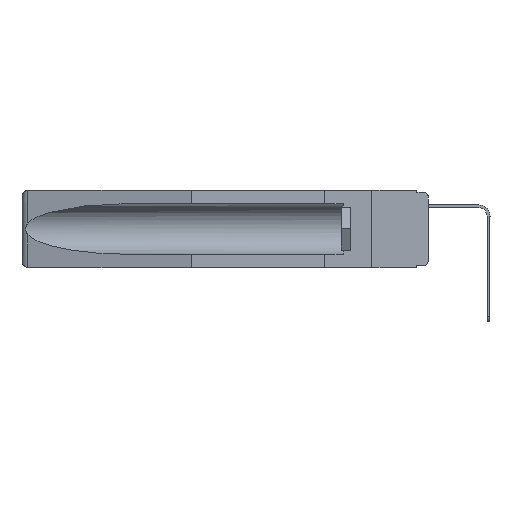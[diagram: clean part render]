
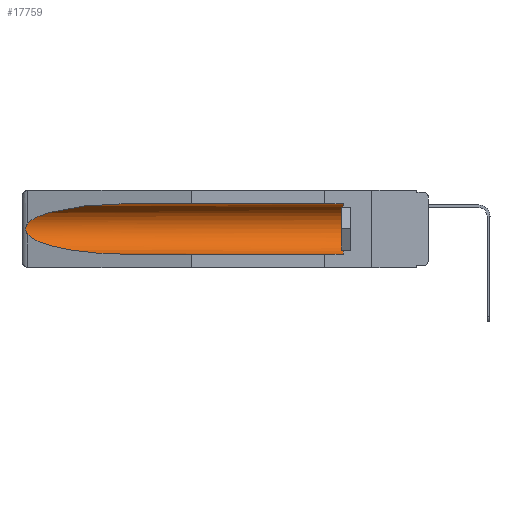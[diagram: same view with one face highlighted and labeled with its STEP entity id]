
A CAD part, left-side view. The second image highlights one B-rep face of the part: STEP entity #17759.
In plain terms, the highlighted cylindrical face has radius 2.857 mm (diameter 5.715 mm), a partial arc.
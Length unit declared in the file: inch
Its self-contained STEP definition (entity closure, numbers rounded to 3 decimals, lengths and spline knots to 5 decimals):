
#1118 = DIRECTION ( 'NONE',  ( 0., 1., 0. ) ) ;
#1183 = CARTESIAN_POINT ( 'NONE',  ( 0.155, 1.07973, -0.059 ) ) ;
#1513 = VERTEX_POINT ( 'NONE', #8068 ) ;
#1855 = CARTESIAN_POINT ( 'NONE',  ( 0.26597, 1.5296, -0.19026 ) ) ;
#2776 = VECTOR ( 'NONE', #13278, 39.37008 ) ;
#3021 = VERTEX_POINT ( 'NONE', #20520 ) ;
#3305 = ORIENTED_EDGE ( 'NONE', *, *, #5859, .T. ) ;
#3402 = EDGE_CURVE ( 'NONE', #7204, #3021, #19782, .T. ) ;
#3507 = ORIENTED_EDGE ( 'NONE', *, *, #18875, .T. ) ;
#3868 = B_SPLINE_CURVE_WITH_KNOTS ( 'NONE', 3,
 ( #24836, #26958, #6157, #8296, #6059, #23250, #27426, #14862, #1855, #10427 ),
 .UNSPECIFIED., .F., .F.,
 ( 4, 2, 2, 2, 4 ),
 ( 0., 0.00029, 0.00058, 0.00087, 0.00117 ),
 .UNSPECIFIED. ) ;
#4509 = ORIENTED_EDGE ( 'NONE', *, *, #27512, .T. ) ;
#4708 = DIRECTION ( 'NONE',  ( 0., 0., 1. ) ) ;
#5330 = CARTESIAN_POINT ( 'NONE',  ( 0.155, 0.126, -0.284 ) ) ;
#5704 = CIRCLE ( 'NONE', #19511, 0.1125 ) ;
#5859 = EDGE_CURVE ( 'NONE', #1513, #5870, #18946, .T. ) ;
#5870 = VERTEX_POINT ( 'NONE', #7346 ) ;
#6059 = CARTESIAN_POINT ( 'NONE',  ( 0.2675, 1.53308, -0.16763 ) ) ;
#6157 = CARTESIAN_POINT ( 'NONE',  ( 0.26654, 1.53092, -0.15636 ) ) ;
#6192 = CARTESIAN_POINT ( 'NONE',  ( 0.155, 0.126, -0.1715 ) ) ;
#7081 = CARTESIAN_POINT ( 'NONE',  ( 0.155, -0.30754, -0.059 ) ) ;
#7204 = VERTEX_POINT ( 'NONE', #5330 ) ;
#7346 = CARTESIAN_POINT ( 'NONE',  ( 0.155, 1.07973, -0.059 ) ) ;
#7823 = FACE_OUTER_BOUND ( 'NONE', #17874, .T. ) ;
#8056 = EDGE_CURVE ( 'NONE', #16991, #3021, #19513, .T. ) ;
#8068 = CARTESIAN_POINT ( 'NONE',  ( 0.155, 0.126, -0.059 ) ) ;
#8178 = ORIENTED_EDGE ( 'NONE', *, *, #3402, .F. ) ;
#8296 = CARTESIAN_POINT ( 'NONE',  ( 0.2673, 1.5327, -0.16383 ) ) ;
#8927 = CARTESIAN_POINT ( 'NONE',  ( 0.155, -0.30754, -0.284 ) ) ;
#9131 = CARTESIAN_POINT ( 'NONE',  ( 0.26537, 1.52718, -0.19328 ) ) ;
#9676 =( BOUNDED_CURVE ( )  B_SPLINE_CURVE ( 3, ( #1183, #18191, #14009, #15885 ),
 .UNSPECIFIED., .F., .F. ) 
 B_SPLINE_CURVE_WITH_KNOTS ( ( 4, 4 ),
 ( 4.71239, 6.08839 ),
 .UNSPECIFIED. ) 
 CURVE ( )  GEOMETRIC_REPRESENTATION_ITEM ( )  RATIONAL_B_SPLINE_CURVE ( ( 1., 0.848, 0.848, 1. ) ) 
 REPRESENTATION_ITEM ( '' )  );
#10427 = CARTESIAN_POINT ( 'NONE',  ( 0.26537, 1.52718, -0.19328 ) ) ;
#10645 = DIRECTION ( 'NONE',  ( 0., 0., 1. ) ) ;
#12142 = CARTESIAN_POINT ( 'NONE',  ( 0.21114, 1.30732, -0.284 ) ) ;
#12329 = CARTESIAN_POINT ( 'NONE',  ( 0.155, 1.07973, -0.284 ) ) ;
#12703 = AXIS2_PLACEMENT_3D ( 'NONE', #17540, #19623, #4708 ) ;
#13278 = DIRECTION ( 'NONE',  ( 0., 1., 0. ) ) ;
#14009 = CARTESIAN_POINT ( 'NONE',  ( 0.25451, 1.48313, -0.09465 ) ) ;
#14862 = CARTESIAN_POINT ( 'NONE',  ( 0.26655, 1.53094, -0.18657 ) ) ;
#15253 = VERTEX_POINT ( 'NONE', #16041 ) ;
#15885 = CARTESIAN_POINT ( 'NONE',  ( 0.26537, 1.52718, -0.14972 ) ) ;
#16041 = CARTESIAN_POINT ( 'NONE',  ( 0.26537, 1.52718, -0.14972 ) ) ;
#16568 = CARTESIAN_POINT ( 'NONE',  ( 0.25451, 1.48313, -0.24835 ) ) ;
#16991 = VERTEX_POINT ( 'NONE', #9131 ) ;
#17540 = CARTESIAN_POINT ( 'NONE',  ( 0.155, -0.30754, -0.1715 ) ) ;
#17759 = ADVANCED_FACE ( 'NONE', ( #7823 ), #24127, .F. ) ;
#17874 = EDGE_LOOP ( 'NONE', ( #23594, #3507, #20569, #8178, #4509, #3305 ) ) ;
#18191 = CARTESIAN_POINT ( 'NONE',  ( 0.21114, 1.30732, -0.059 ) ) ;
#18875 = EDGE_CURVE ( 'NONE', #15253, #16991, #3868, .T. ) ;
#18946 = LINE ( 'NONE', #7081, #22821 ) ;
#19285 = EDGE_CURVE ( 'NONE', #5870, #15253, #9676, .T. ) ;
#19511 = AXIS2_PLACEMENT_3D ( 'NONE', #6192, #21068, #10645 ) ;
#19513 =( BOUNDED_CURVE ( )  B_SPLINE_CURVE ( 3, ( #20690, #16568, #12142, #12329 ),
 .UNSPECIFIED., .F., .F. ) 
 B_SPLINE_CURVE_WITH_KNOTS ( ( 4, 4 ),
 ( 0.1948, 1.5708 ),
 .UNSPECIFIED. ) 
 CURVE ( )  GEOMETRIC_REPRESENTATION_ITEM ( )  RATIONAL_B_SPLINE_CURVE ( ( 1., 0.848, 0.848, 1. ) ) 
 REPRESENTATION_ITEM ( '' )  );
#19623 = DIRECTION ( 'NONE',  ( 0., 1., 0. ) ) ;
#19782 = LINE ( 'NONE', #8927, #2776 ) ;
#20520 = CARTESIAN_POINT ( 'NONE',  ( 0.155, 1.07973, -0.284 ) ) ;
#20569 = ORIENTED_EDGE ( 'NONE', *, *, #8056, .T. ) ;
#20690 = CARTESIAN_POINT ( 'NONE',  ( 0.26537, 1.52718, -0.19328 ) ) ;
#21068 = DIRECTION ( 'NONE',  ( 0., -1., 0. ) ) ;
#22821 = VECTOR ( 'NONE', #1118, 39.37008 ) ;
#23250 = CARTESIAN_POINT ( 'NONE',  ( 0.2675, 1.53308, -0.17534 ) ) ;
#23594 = ORIENTED_EDGE ( 'NONE', *, *, #19285, .T. ) ;
#24127 = CYLINDRICAL_SURFACE ( 'NONE', #12703, 0.1125 ) ;
#24836 = CARTESIAN_POINT ( 'NONE',  ( 0.26537, 1.52718, -0.14972 ) ) ;
#26958 = CARTESIAN_POINT ( 'NONE',  ( 0.26597, 1.52961, -0.15275 ) ) ;
#27426 = CARTESIAN_POINT ( 'NONE',  ( 0.2673, 1.53269, -0.17917 ) ) ;
#27512 = EDGE_CURVE ( 'NONE', #7204, #1513, #5704, .T. ) ;
